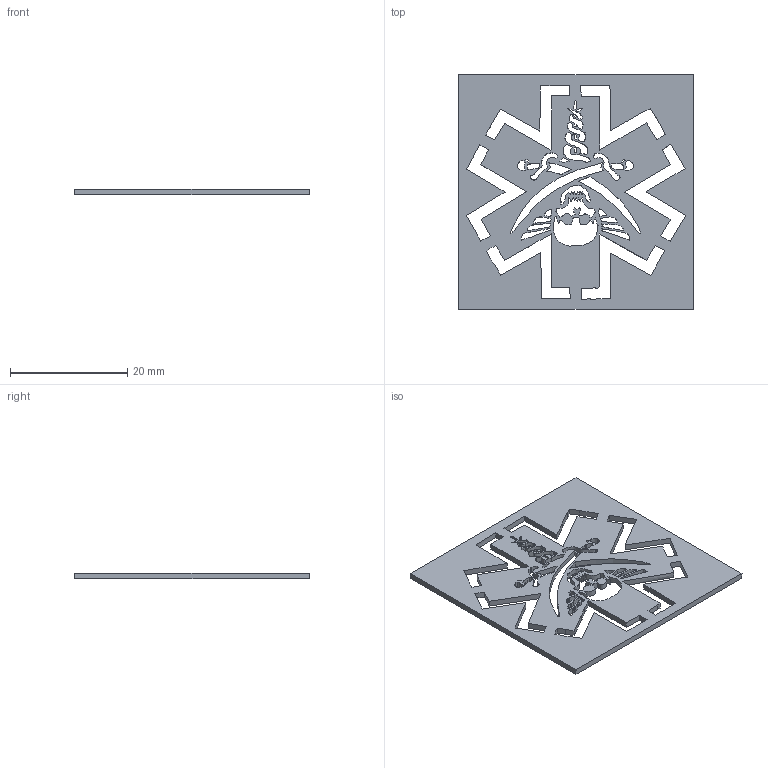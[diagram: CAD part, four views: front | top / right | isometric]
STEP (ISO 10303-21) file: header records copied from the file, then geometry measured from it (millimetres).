
FILE_DESCRIPTION (( 'STEP AP214' ), '1' );
FILE_NAME ('Pirate_Medic.STEP', '2013-09-01T16:53:40', ( 'Asher' ), ( '' ), 'SwSTEP 2.0', 'SolidWorks 2013', '' );
FILE_SCHEMA (( 'AUTOMOTIVE_DESIGN' ));
Length unit declared in the file: millimetre
Products named in the file (1): Pirate_Medic
Bounding box: 40 x 40 x 1 mm (x, y, z)
Volume: 1176.3 mm3; surface area: 3190.8 mm2
Topology: 1 solids, 1 shells, 403 faces, 1203 edges, 802 vertices
Faces by surface type: plane 303, bspline 100
Entity records: 16883 total; most frequent: CARTESIAN_POINT 6549, ORIENTED_EDGE 2406, DIRECTION 1611, EDGE_CURVE 1203, VECTOR 1003, LINE 1003, VERTEX_POINT 802, EDGE_LOOP 479
